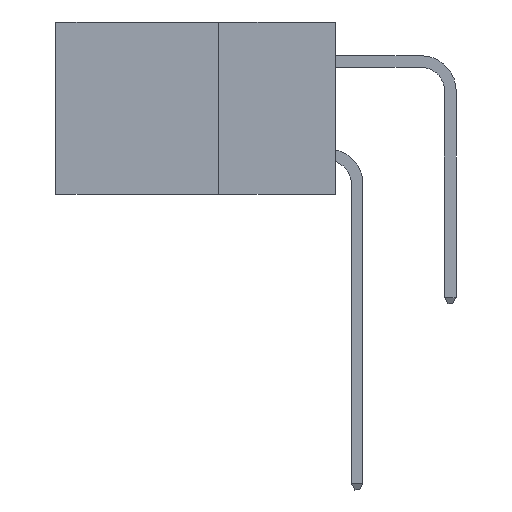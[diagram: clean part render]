
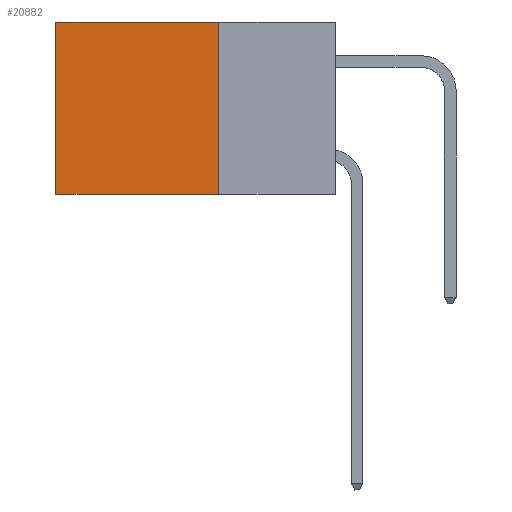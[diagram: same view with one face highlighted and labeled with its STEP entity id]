
A CAD part, left-side view. The second image highlights one B-rep face of the part: STEP entity #20882.
In plain terms, the highlighted planar face has unit normal (-1, 0, 0).
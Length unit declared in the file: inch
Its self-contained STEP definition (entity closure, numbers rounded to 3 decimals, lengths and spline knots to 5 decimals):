
#933 = LINE ( 'NONE', #7585, #15866 ) ;
#1798 = CARTESIAN_POINT ( 'NONE',  ( 0.2875, 0.6, -0.37 ) ) ;
#2302 = DIRECTION ( 'NONE',  ( 0., 0., -1. ) ) ;
#2802 = AXIS2_PLACEMENT_3D ( 'NONE', #10691, #21508, #2302 ) ;
#4045 = VERTEX_POINT ( 'NONE', #15939 ) ;
#4651 = FACE_OUTER_BOUND ( 'NONE', #7189, .T. ) ;
#4733 = VECTOR ( 'NONE', #18355, 39.37008 ) ;
#6235 = PLANE ( 'NONE',  #2802 ) ;
#6537 = CARTESIAN_POINT ( 'NONE',  ( 0.2875, 0.6, 0. ) ) ;
#7134 = VECTOR ( 'NONE', #21201, 39.37008 ) ;
#7189 = EDGE_LOOP ( 'NONE', ( #19060, #22657, #15251, #22998 ) ) ;
#7446 = CARTESIAN_POINT ( 'NONE',  ( 0.2875, 0.25, 0. ) ) ;
#7585 = CARTESIAN_POINT ( 'NONE',  ( 0.2875, 0.25, -0.37 ) ) ;
#8356 = LINE ( 'NONE', #6537, #10082 ) ;
#8689 = DIRECTION ( 'NONE',  ( 0., 0., -1. ) ) ;
#9087 = VERTEX_POINT ( 'NONE', #25389 ) ;
#9983 = CARTESIAN_POINT ( 'NONE',  ( 0.2875, 0.25, 0. ) ) ;
#10082 = VECTOR ( 'NONE', #8689, 39.37008 ) ;
#10691 = CARTESIAN_POINT ( 'NONE',  ( 0.2875, 0.25, 0. ) ) ;
#12249 = LINE ( 'NONE', #21110, #7134 ) ;
#12775 = VERTEX_POINT ( 'NONE', #9983 ) ;
#13534 = EDGE_CURVE ( 'NONE', #9087, #18383, #8356, .T. ) ;
#15251 = ORIENTED_EDGE ( 'NONE', *, *, #23897, .F. ) ;
#15866 = VECTOR ( 'NONE', #24874, 39.37008 ) ;
#15939 = CARTESIAN_POINT ( 'NONE',  ( 0.2875, 0.25, -0.37 ) ) ;
#18355 = DIRECTION ( 'NONE',  ( 0., 1., 0. ) ) ;
#18383 = VERTEX_POINT ( 'NONE', #1798 ) ;
#19060 = ORIENTED_EDGE ( 'NONE', *, *, #13534, .T. ) ;
#20882 = ADVANCED_FACE ( 'NONE', ( #4651 ), #6235, .F. ) ;
#21110 = CARTESIAN_POINT ( 'NONE',  ( 0.2875, 0.25, 0. ) ) ;
#21201 = DIRECTION ( 'NONE',  ( 0., 0., -1. ) ) ;
#21508 = DIRECTION ( 'NONE',  ( 1., 0., 0. ) ) ;
#22657 = ORIENTED_EDGE ( 'NONE', *, *, #26101, .F. ) ;
#22998 = ORIENTED_EDGE ( 'NONE', *, *, #25556, .T. ) ;
#23455 = LINE ( 'NONE', #7446, #4733 ) ;
#23897 = EDGE_CURVE ( 'NONE', #12775, #4045, #12249, .T. ) ;
#24874 = DIRECTION ( 'NONE',  ( 0., 1., 0. ) ) ;
#25389 = CARTESIAN_POINT ( 'NONE',  ( 0.2875, 0.6, 0. ) ) ;
#25556 = EDGE_CURVE ( 'NONE', #12775, #9087, #23455, .T. ) ;
#26101 = EDGE_CURVE ( 'NONE', #4045, #18383, #933, .T. ) ;
